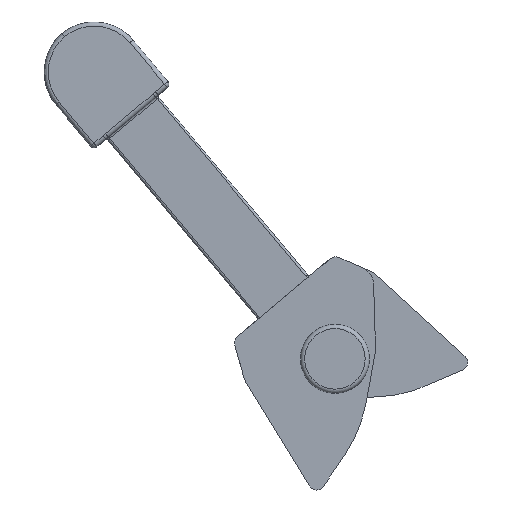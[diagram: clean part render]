
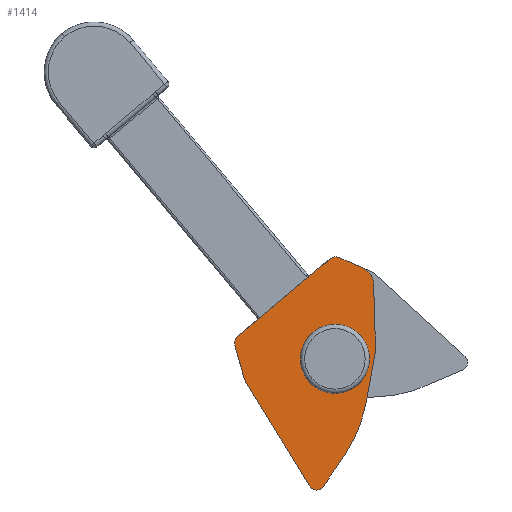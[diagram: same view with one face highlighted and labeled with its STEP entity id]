
A CAD part, left-side view. The second image highlights one B-rep face of the part: STEP entity #1414.
In plain terms, the highlighted planar face has unit normal (-1, 0, 0).
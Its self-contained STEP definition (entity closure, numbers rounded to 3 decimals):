
#16=FACE_BOUND('',#252,.T.);
#82=PLANE('',#1593);
#163=FACE_OUTER_BOUND('',#251,.T.);
#251=EDGE_LOOP('',(#1224,#1225,#1226,#1227,#1228,#1229,#1230,#1231,#1232,
#1233,#1234,#1235,#1236,#1237));
#252=EDGE_LOOP('',(#1238));
#275=LINE('',#2092,#375);
#281=LINE('',#2113,#381);
#286=LINE('',#2125,#386);
#298=LINE('',#2158,#398);
#346=LINE('',#2746,#446);
#353=LINE('',#2761,#453);
#357=LINE('',#2769,#457);
#375=VECTOR('',#1641,10.);
#381=VECTOR('',#1659,10.);
#386=VECTOR('',#1670,10.);
#398=VECTOR('',#1698,10.);
#446=VECTOR('',#1984,10.);
#453=VECTOR('',#2001,10.);
#457=VECTOR('',#2011,10.);
#469=CIRCLE('',#1447,1.);
#474=CIRCLE('',#1456,16.);
#475=CIRCLE('',#1459,1.);
#489=CIRCLE('',#1480,4.06);
#542=CIRCLE('',#1588,2.);
#543=CIRCLE('',#1591,2.);
#544=CIRCLE('',#1594,1.);
#545=CIRCLE('',#1595,1.);
#560=VERTEX_POINT('',#2082);
#561=VERTEX_POINT('',#2084);
#563=VERTEX_POINT('',#2090);
#572=VERTEX_POINT('',#2112);
#573=VERTEX_POINT('',#2116);
#575=VERTEX_POINT('',#2122);
#576=VERTEX_POINT('',#2124);
#586=VERTEX_POINT('',#2150);
#589=VERTEX_POINT('',#2156);
#597=VERTEX_POINT('',#2181);
#666=VERTEX_POINT('',#2742);
#668=VERTEX_POINT('',#2745);
#670=VERTEX_POINT('',#2756);
#671=VERTEX_POINT('',#2760);
#672=VERTEX_POINT('',#2764);
#687=EDGE_CURVE('',#561,#560,#469,.T.);
#691=EDGE_CURVE('',#560,#563,#275,.T.);
#701=EDGE_CURVE('',#572,#561,#281,.T.);
#704=EDGE_CURVE('',#563,#573,#474,.T.);
#707=EDGE_CURVE('',#576,#575,#286,.T.);
#710=EDGE_CURVE('',#575,#572,#475,.T.);
#724=EDGE_CURVE('',#586,#589,#298,.T.);
#735=EDGE_CURVE('',#597,#597,#489,.T.);
#856=EDGE_CURVE('',#668,#666,#346,.T.);
#862=EDGE_CURVE('',#670,#586,#542,.T.);
#864=EDGE_CURVE('',#671,#670,#353,.T.);
#866=EDGE_CURVE('',#672,#671,#543,.T.);
#869=EDGE_CURVE('',#573,#672,#357,.T.);
#870=EDGE_CURVE('',#589,#668,#544,.T.);
#871=EDGE_CURVE('',#666,#576,#545,.T.);
#1224=ORIENTED_EDGE('',*,*,#704,.T.);
#1225=ORIENTED_EDGE('',*,*,#869,.T.);
#1226=ORIENTED_EDGE('',*,*,#866,.T.);
#1227=ORIENTED_EDGE('',*,*,#864,.T.);
#1228=ORIENTED_EDGE('',*,*,#862,.T.);
#1229=ORIENTED_EDGE('',*,*,#724,.T.);
#1230=ORIENTED_EDGE('',*,*,#870,.T.);
#1231=ORIENTED_EDGE('',*,*,#856,.T.);
#1232=ORIENTED_EDGE('',*,*,#871,.T.);
#1233=ORIENTED_EDGE('',*,*,#707,.T.);
#1234=ORIENTED_EDGE('',*,*,#710,.T.);
#1235=ORIENTED_EDGE('',*,*,#701,.T.);
#1236=ORIENTED_EDGE('',*,*,#687,.T.);
#1237=ORIENTED_EDGE('',*,*,#691,.T.);
#1238=ORIENTED_EDGE('',*,*,#735,.F.);
#1414=ADVANCED_FACE('',(#163,#16),#82,.F.);
#1447=AXIS2_PLACEMENT_3D('',#2085,#1634,#1635);
#1456=AXIS2_PLACEMENT_3D('',#2118,#1664,#1665);
#1459=AXIS2_PLACEMENT_3D('',#2130,#1675,#1676);
#1480=AXIS2_PLACEMENT_3D('',#2182,#1728,#1729);
#1588=AXIS2_PLACEMENT_3D('',#2757,#1996,#1997);
#1591=AXIS2_PLACEMENT_3D('',#2765,#2005,#2006);
#1593=AXIS2_PLACEMENT_3D('',#2770,#2012,#2013);
#1594=AXIS2_PLACEMENT_3D('',#2771,#2014,#2015);
#1595=AXIS2_PLACEMENT_3D('',#2772,#2016,#2017);
#1634=DIRECTION('center_axis',(-1.,0.,0.));
#1635=DIRECTION('ref_axis',(0.,0.853,-0.521));
#1641=DIRECTION('',(0.,-0.558,0.83));
#1659=DIRECTION('',(0.,-0.521,-0.853));
#1664=DIRECTION('center_axis',(-1.,0.,0.));
#1665=DIRECTION('ref_axis',(0.,-0.983,-0.182));
#1670=DIRECTION('',(0.,-0.276,-0.961));
#1675=DIRECTION('center_axis',(-1.,0.,0.));
#1676=DIRECTION('ref_axis',(0.,0.853,-0.521));
#1698=DIRECTION('',(0.,0.918,0.398));
#1728=DIRECTION('center_axis',(-1.,0.,0.));
#1729=DIRECTION('ref_axis',(0.,0.766,-0.643));
#1984=DIRECTION('',(0.,0.766,-0.643));
#1996=DIRECTION('center_axis',(-1.,0.,0.));
#1997=DIRECTION('ref_axis',(0.,-0.398,0.918));
#2001=DIRECTION('',(0.,0.029,1.));
#2005=DIRECTION('center_axis',(-1.,0.,0.));
#2006=DIRECTION('ref_axis',(0.,-1.,0.029));
#2011=DIRECTION('',(0.,-0.182,0.983));
#2012=DIRECTION('center_axis',(1.,0.,0.));
#2013=DIRECTION('ref_axis',(0.,0.766,-0.643));
#2014=DIRECTION('center_axis',(-1.,0.,0.));
#2015=DIRECTION('ref_axis',(0.,0.643,0.766));
#2016=DIRECTION('center_axis',(-1.,0.,0.));
#2017=DIRECTION('ref_axis',(0.,0.961,-0.276));
#2082=CARTESIAN_POINT('',(-108.968,-9.753,15.277));
#2084=CARTESIAN_POINT('',(-108.968,-8.07,15.314));
#2085=CARTESIAN_POINT('Origin',(-108.968,-8.923,15.835));
#2090=CARTESIAN_POINT('',(-108.968,-12.279,19.034));
#2092=CARTESIAN_POINT('',(-108.968,-9.753,15.277));
#2112=CARTESIAN_POINT('',(-108.968,-0.544,27.638));
#2113=CARTESIAN_POINT('',(-108.968,-0.544,27.638));
#2116=CARTESIAN_POINT('',(-108.968,-14.733,25.045));
#2118=CARTESIAN_POINT('Origin',(-108.968,0.999,27.961));
#2122=CARTESIAN_POINT('',(-108.968,-0.437,27.883));
#2124=CARTESIAN_POINT('',(-108.968,0.707,31.861));
#2125=CARTESIAN_POINT('',(-108.968,-0.437,27.883));
#2130=CARTESIAN_POINT('Origin',(-108.968,-1.398,28.159));
#2150=CARTESIAN_POINT('',(-108.968,-14.437,40.954));
#2156=CARTESIAN_POINT('',(-108.968,-11.554,42.203));
#2158=CARTESIAN_POINT('',(-108.968,-11.554,42.203));
#2181=CARTESIAN_POINT('',(-108.968,-14.198,32.881));
#2182=CARTESIAN_POINT('Origin',(-108.968,-11.088,30.271));
#2742=CARTESIAN_POINT('',(-108.968,0.389,32.903));
#2745=CARTESIAN_POINT('',(-108.968,-10.514,42.052));
#2746=CARTESIAN_POINT('',(-108.968,0.887,32.486));
#2756=CARTESIAN_POINT('',(-108.968,-15.64,39.177));
#2757=CARTESIAN_POINT('Origin',(-108.968,-13.641,39.119));
#2760=CARTESIAN_POINT('',(-108.968,-15.867,31.409));
#2761=CARTESIAN_POINT('',(-108.968,-15.867,31.409));
#2764=CARTESIAN_POINT('',(-108.968,-15.834,30.986));
#2765=CARTESIAN_POINT('Origin',(-108.968,-13.867,31.351));
#2769=CARTESIAN_POINT('',(-108.968,-14.733,25.045));
#2770=CARTESIAN_POINT('Origin',(-108.968,-10.472,29.361));
#2771=CARTESIAN_POINT('Origin',(-108.968,-11.157,41.286));
#2772=CARTESIAN_POINT('Origin',(-108.968,-0.254,32.137));
